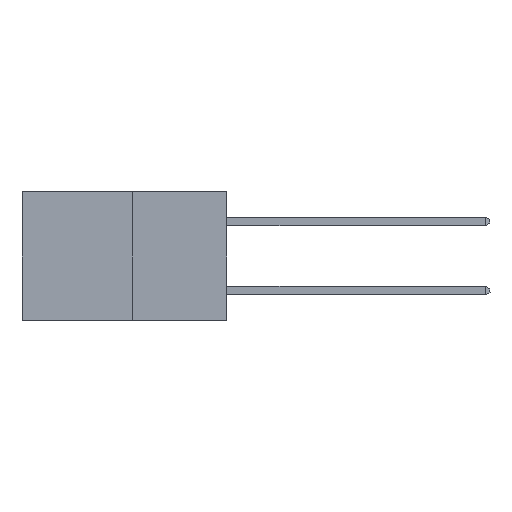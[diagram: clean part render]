
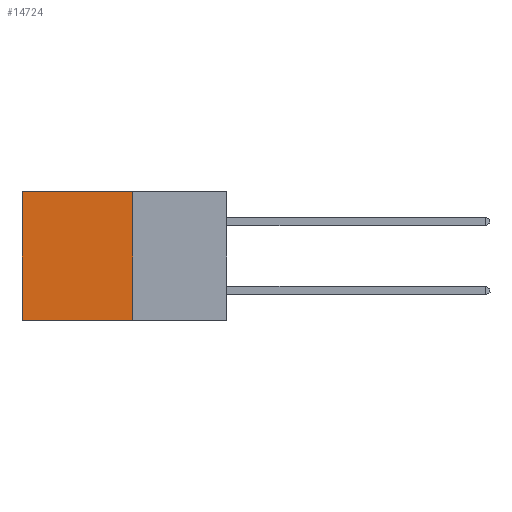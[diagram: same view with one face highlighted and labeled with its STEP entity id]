
A CAD part, left-side view. The second image highlights one B-rep face of the part: STEP entity #14724.
In plain terms, the highlighted planar face has unit normal (-1, 0, 0).
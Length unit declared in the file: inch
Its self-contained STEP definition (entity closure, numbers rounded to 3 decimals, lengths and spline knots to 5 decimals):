
#588 = LINE ( 'NONE', #3594, #20773 ) ;
#700 = CARTESIAN_POINT ( 'NONE',  ( 0.277, 0.27, -0.37 ) ) ;
#918 = DIRECTION ( 'NONE',  ( 0., 0., -1. ) ) ;
#1556 = ORIENTED_EDGE ( 'NONE', *, *, #5689, .T. ) ;
#1819 = PLANE ( 'NONE',  #3713 ) ;
#2714 = ORIENTED_EDGE ( 'NONE', *, *, #3598, .F. ) ;
#3594 = CARTESIAN_POINT ( 'NONE',  ( 0.277, 0.27, -0.37 ) ) ;
#3598 = EDGE_CURVE ( 'NONE', #12963, #22840, #588, .T. ) ;
#3713 = AXIS2_PLACEMENT_3D ( 'NONE', #12414, #20216, #4510 ) ;
#4037 = CARTESIAN_POINT ( 'NONE',  ( 0.277, 0.27, 0. ) ) ;
#4510 = DIRECTION ( 'NONE',  ( 0., 0., -1. ) ) ;
#4974 = DIRECTION ( 'NONE',  ( 0., 1., 0. ) ) ;
#5169 = CARTESIAN_POINT ( 'NONE',  ( 0.277, 0.27, -0.37 ) ) ;
#5210 = LINE ( 'NONE', #23179, #31892 ) ;
#5689 = EDGE_CURVE ( 'NONE', #11563, #31518, #18135, .T. ) ;
#6307 = DIRECTION ( 'NONE',  ( 0., 0., -1. ) ) ;
#7860 = ORIENTED_EDGE ( 'NONE', *, *, #33488, .T. ) ;
#8862 = EDGE_CURVE ( 'NONE', #22840, #31518, #10986, .T. ) ;
#10157 = VECTOR ( 'NONE', #26809, 39.37008 ) ;
#10421 = VECTOR ( 'NONE', #918, 39.37008 ) ;
#10986 = LINE ( 'NONE', #700, #10157 ) ;
#11563 = VERTEX_POINT ( 'NONE', #16787 ) ;
#12414 = CARTESIAN_POINT ( 'NONE',  ( 0.277, 0.27, -0.37 ) ) ;
#12963 = VERTEX_POINT ( 'NONE', #4037 ) ;
#13929 = CARTESIAN_POINT ( 'NONE',  ( 0.277, 0.59, -0.37 ) ) ;
#14724 = ADVANCED_FACE ( 'NONE', ( #19408 ), #1819, .F. ) ;
#16787 = CARTESIAN_POINT ( 'NONE',  ( 0.277, 0.59, 0. ) ) ;
#18135 = LINE ( 'NONE', #19350, #10421 ) ;
#18984 = EDGE_LOOP ( 'NONE', ( #1556, #19133, #2714, #7860 ) ) ;
#19133 = ORIENTED_EDGE ( 'NONE', *, *, #8862, .F. ) ;
#19350 = CARTESIAN_POINT ( 'NONE',  ( 0.277, 0.59, -0.37 ) ) ;
#19408 = FACE_OUTER_BOUND ( 'NONE', #18984, .T. ) ;
#20216 = DIRECTION ( 'NONE',  ( 1., 0., 0. ) ) ;
#20773 = VECTOR ( 'NONE', #6307, 39.37008 ) ;
#22840 = VERTEX_POINT ( 'NONE', #5169 ) ;
#23179 = CARTESIAN_POINT ( 'NONE',  ( 0.277, 0.27, 0. ) ) ;
#26809 = DIRECTION ( 'NONE',  ( 0., 1., 0. ) ) ;
#31518 = VERTEX_POINT ( 'NONE', #13929 ) ;
#31892 = VECTOR ( 'NONE', #4974, 39.37008 ) ;
#33488 = EDGE_CURVE ( 'NONE', #12963, #11563, #5210, .T. ) ;
